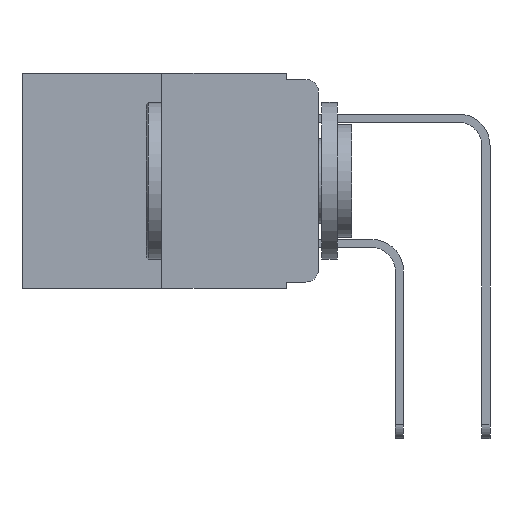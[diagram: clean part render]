
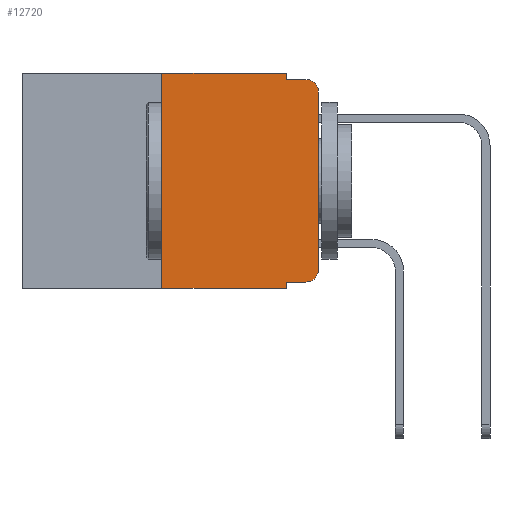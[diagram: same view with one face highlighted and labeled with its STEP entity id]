
A CAD part, left-side view. The second image highlights one B-rep face of the part: STEP entity #12720.
In plain terms, the highlighted planar face has unit normal (-1, 0, 0).
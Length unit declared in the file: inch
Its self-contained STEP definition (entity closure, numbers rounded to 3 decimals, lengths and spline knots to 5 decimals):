
#292 = VECTOR ( 'NONE', #5764, 39.37008 ) ;
#305 = EDGE_CURVE ( 'NONE', #5606, #10131, #492, .T. ) ;
#492 = LINE ( 'NONE', #9587, #11351 ) ;
#646 = DIRECTION ( 'NONE',  ( 0., 0., -1. ) ) ;
#768 = CARTESIAN_POINT ( 'NONE',  ( 0., 0.051, 0. ) ) ;
#880 = VERTEX_POINT ( 'NONE', #5435 ) ;
#1061 = ORIENTED_EDGE ( 'NONE', *, *, #11366, .T. ) ;
#1077 = CARTESIAN_POINT ( 'NONE',  ( 0., 0.25, 0. ) ) ;
#1200 = EDGE_CURVE ( 'NONE', #4556, #8043, #4459, .T. ) ;
#1260 = FACE_OUTER_BOUND ( 'NONE', #11446, .T. ) ;
#1419 = ORIENTED_EDGE ( 'NONE', *, *, #1200, .F. ) ;
#1617 = CARTESIAN_POINT ( 'NONE',  ( 0., 0.051, -0.01 ) ) ;
#1693 = VECTOR ( 'NONE', #9176, 39.37008 ) ;
#1787 = LINE ( 'NONE', #1077, #12738 ) ;
#1972 = AXIS2_PLACEMENT_3D ( 'NONE', #9889, #3657, #10889 ) ;
#2123 = CIRCLE ( 'NONE', #1972, 0.02 ) ;
#2183 = CARTESIAN_POINT ( 'NONE',  ( 0., 0.051, 0. ) ) ;
#2469 = CARTESIAN_POINT ( 'NONE',  ( 0., 0.051, -0.01 ) ) ;
#2500 = EDGE_CURVE ( 'NONE', #2912, #3912, #4597, .T. ) ;
#2856 = VERTEX_POINT ( 'NONE', #9729 ) ;
#2912 = VERTEX_POINT ( 'NONE', #7145 ) ;
#3136 = ORIENTED_EDGE ( 'NONE', *, *, #2500, .T. ) ;
#3233 = CARTESIAN_POINT ( 'NONE',  ( 0., 0.25, 0. ) ) ;
#3252 = LINE ( 'NONE', #8854, #292 ) ;
#3411 = VERTEX_POINT ( 'NONE', #10804 ) ;
#3655 = DIRECTION ( 'NONE',  ( 0., 0., 1. ) ) ;
#3657 = DIRECTION ( 'NONE',  ( -1., 0., 0. ) ) ;
#3660 = CARTESIAN_POINT ( 'NONE',  ( 0., 0., -0.03 ) ) ;
#3769 = VECTOR ( 'NONE', #6990, 39.37008 ) ;
#3844 = ORIENTED_EDGE ( 'NONE', *, *, #7596, .T. ) ;
#3912 = VERTEX_POINT ( 'NONE', #10260 ) ;
#4110 = DIRECTION ( 'NONE',  ( 0., 0., -1. ) ) ;
#4194 = ORIENTED_EDGE ( 'NONE', *, *, #12873, .T. ) ;
#4459 = LINE ( 'NONE', #2469, #3769 ) ;
#4556 = VERTEX_POINT ( 'NONE', #1617 ) ;
#4597 = LINE ( 'NONE', #12189, #1693 ) ;
#4783 = EDGE_CURVE ( 'NONE', #880, #6468, #5180, .T. ) ;
#5180 = LINE ( 'NONE', #7644, #10340 ) ;
#5435 = CARTESIAN_POINT ( 'NONE',  ( 0., 0., -0.313 ) ) ;
#5439 = CARTESIAN_POINT ( 'NONE',  ( 0., 0.02, -0.01 ) ) ;
#5519 = DIRECTION ( 'NONE',  ( 1., 0., 0. ) ) ;
#5606 = VERTEX_POINT ( 'NONE', #3233 ) ;
#5764 = DIRECTION ( 'NONE',  ( 0., -1., 0. ) ) ;
#6140 = ORIENTED_EDGE ( 'NONE', *, *, #4783, .T. ) ;
#6468 = VERTEX_POINT ( 'NONE', #3660 ) ;
#6710 = DIRECTION ( 'NONE',  ( 0., 0., -1. ) ) ;
#6990 = DIRECTION ( 'NONE',  ( 0., -1., 0. ) ) ;
#6997 = EDGE_CURVE ( 'NONE', #10131, #4556, #12829, .T. ) ;
#7123 = DIRECTION ( 'NONE',  ( -1., 0., 0. ) ) ;
#7145 = CARTESIAN_POINT ( 'NONE',  ( 0., 0.25, -0.343 ) ) ;
#7585 = VECTOR ( 'NONE', #6710, 39.37008 ) ;
#7593 = PLANE ( 'NONE',  #11949 ) ;
#7596 = EDGE_CURVE ( 'NONE', #3411, #2856, #3252, .T. ) ;
#7644 = CARTESIAN_POINT ( 'NONE',  ( 0., 0., 0. ) ) ;
#7758 = CARTESIAN_POINT ( 'NONE',  ( 0., 0.051, 0. ) ) ;
#7891 = VECTOR ( 'NONE', #4110, 39.37008 ) ;
#8043 = VERTEX_POINT ( 'NONE', #5439 ) ;
#8548 = DIRECTION ( 'NONE',  ( 0., 0., 1. ) ) ;
#8764 = EDGE_CURVE ( 'NONE', #3411, #3912, #10589, .T. ) ;
#8854 = CARTESIAN_POINT ( 'NONE',  ( 0., 0.051, -0.333 ) ) ;
#9176 = DIRECTION ( 'NONE',  ( 0., -1., 0. ) ) ;
#9587 = CARTESIAN_POINT ( 'NONE',  ( 0., 0.473, 0. ) ) ;
#9729 = CARTESIAN_POINT ( 'NONE',  ( 0., 0.02, -0.333 ) ) ;
#9772 = CIRCLE ( 'NONE', #12101, 0.02 ) ;
#9889 = CARTESIAN_POINT ( 'NONE',  ( 0., 0.02, -0.313 ) ) ;
#10131 = VERTEX_POINT ( 'NONE', #2183 ) ;
#10260 = CARTESIAN_POINT ( 'NONE',  ( 0., 0.051, -0.343 ) ) ;
#10340 = VECTOR ( 'NONE', #3655, 39.37008 ) ;
#10589 = LINE ( 'NONE', #768, #7891 ) ;
#10804 = CARTESIAN_POINT ( 'NONE',  ( 0., 0.051, -0.333 ) ) ;
#10889 = DIRECTION ( 'NONE',  ( 0., 0., -1. ) ) ;
#11351 = VECTOR ( 'NONE', #11804, 39.37008 ) ;
#11366 = EDGE_CURVE ( 'NONE', #6468, #8043, #9772, .T. ) ;
#11446 = EDGE_LOOP ( 'NONE', ( #6140, #1061, #1419, #12439, #13023, #13300, #3136, #11692, #3844, #4194 ) ) ;
#11604 = CARTESIAN_POINT ( 'NONE',  ( 0., 0.473, 0. ) ) ;
#11692 = ORIENTED_EDGE ( 'NONE', *, *, #8764, .F. ) ;
#11804 = DIRECTION ( 'NONE',  ( 0., -1., 0. ) ) ;
#11949 = AXIS2_PLACEMENT_3D ( 'NONE', #11604, #5519, #12571 ) ;
#12101 = AXIS2_PLACEMENT_3D ( 'NONE', #13051, #7123, #646 ) ;
#12189 = CARTESIAN_POINT ( 'NONE',  ( 0., 0.473, -0.343 ) ) ;
#12439 = ORIENTED_EDGE ( 'NONE', *, *, #6997, .F. ) ;
#12571 = DIRECTION ( 'NONE',  ( 0., 0., -1. ) ) ;
#12720 = ADVANCED_FACE ( 'NONE', ( #1260 ), #7593, .F. ) ;
#12738 = VECTOR ( 'NONE', #8548, 39.37008 ) ;
#12829 = LINE ( 'NONE', #7758, #7585 ) ;
#12873 = EDGE_CURVE ( 'NONE', #2856, #880, #2123, .T. ) ;
#13023 = ORIENTED_EDGE ( 'NONE', *, *, #305, .F. ) ;
#13051 = CARTESIAN_POINT ( 'NONE',  ( 0., 0.02, -0.03 ) ) ;
#13257 = EDGE_CURVE ( 'NONE', #2912, #5606, #1787, .T. ) ;
#13300 = ORIENTED_EDGE ( 'NONE', *, *, #13257, .F. ) ;
